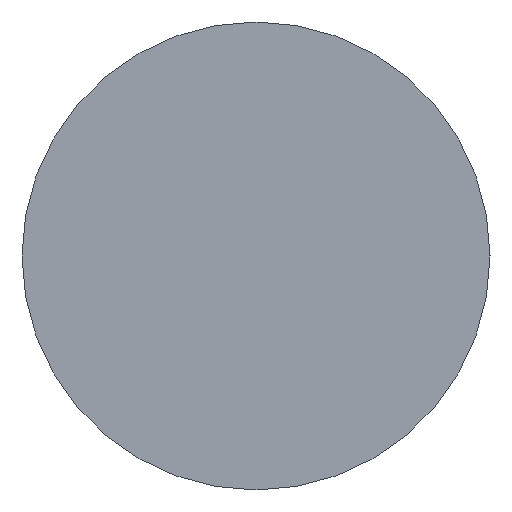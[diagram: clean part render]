
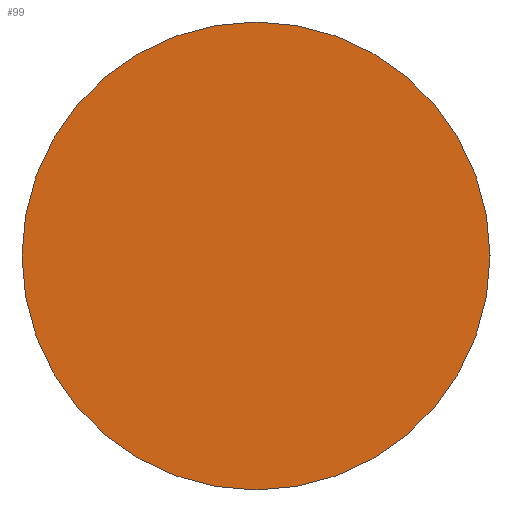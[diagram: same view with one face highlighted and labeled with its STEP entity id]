
A CAD part, left-side view. The second image highlights one B-rep face of the part: STEP entity #99.
In plain terms, the highlighted planar face has unit normal (-1, 0, 0).
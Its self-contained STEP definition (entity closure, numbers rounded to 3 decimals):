
#9 = VERTEX_POINT ( 'NONE', #112 ) ;
#15 = CIRCLE ( 'NONE', #67, 3.75 ) ;
#26 = ORIENTED_EDGE ( 'NONE', *, *, #87, .F. ) ;
#35 = EDGE_LOOP ( 'NONE', ( #109, #26 ) ) ;
#53 = VERTEX_POINT ( 'NONE', #172 ) ;
#64 = AXIS2_PLACEMENT_3D ( 'NONE', #129, #154, #160 ) ;
#67 = AXIS2_PLACEMENT_3D ( 'NONE', #103, #136, #133 ) ;
#79 = AXIS2_PLACEMENT_3D ( 'NONE', #145, #142, #117 ) ;
#87 = EDGE_CURVE ( 'NONE', #9, #53, #107, .T. ) ;
#99 = ADVANCED_FACE ( 'NONE', ( #111 ), #158, .F. ) ;
#103 = CARTESIAN_POINT ( 'NONE',  ( 6.875, 0., 0. ) ) ;
#105 = EDGE_CURVE ( 'NONE', #53, #9, #15, .T. ) ;
#107 = CIRCLE ( 'NONE', #79, 3.75 ) ;
#109 = ORIENTED_EDGE ( 'NONE', *, *, #105, .F. ) ;
#111 = FACE_OUTER_BOUND ( 'NONE', #35, .T. ) ;
#112 = CARTESIAN_POINT ( 'NONE',  ( 6.875, 0., -3.75 ) ) ;
#117 = DIRECTION ( 'NONE',  ( 0., 0., -1. ) ) ;
#129 = CARTESIAN_POINT ( 'NONE',  ( 6.875, 0., 0. ) ) ;
#133 = DIRECTION ( 'NONE',  ( 0., 0., -1. ) ) ;
#136 = DIRECTION ( 'NONE',  ( 1., 0., 0. ) ) ;
#142 = DIRECTION ( 'NONE',  ( 1., 0., 0. ) ) ;
#145 = CARTESIAN_POINT ( 'NONE',  ( 6.875, 0., 0. ) ) ;
#154 = DIRECTION ( 'NONE',  ( 1., 0., 0. ) ) ;
#158 = PLANE ( 'NONE',  #64 ) ;
#160 = DIRECTION ( 'NONE',  ( 0., 0., -1. ) ) ;
#172 = CARTESIAN_POINT ( 'NONE',  ( 6.875, 0., 3.75 ) ) ;
